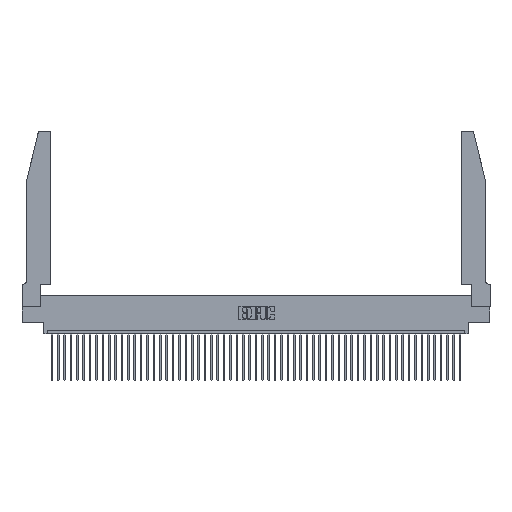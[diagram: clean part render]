
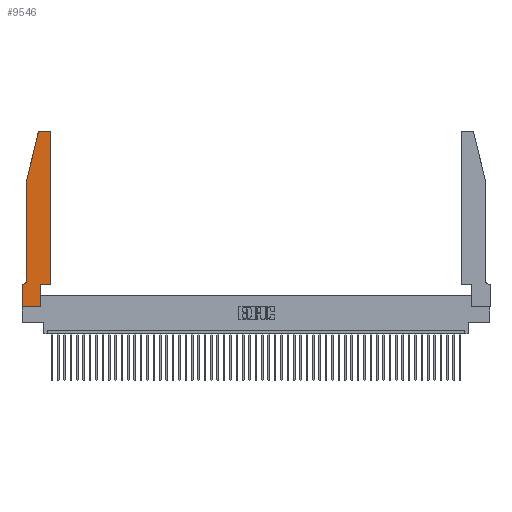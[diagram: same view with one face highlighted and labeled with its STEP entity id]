
A CAD part, top view. The second image highlights one B-rep face of the part: STEP entity #9546.
In plain terms, the highlighted planar face has unit normal (0, 0, 1).
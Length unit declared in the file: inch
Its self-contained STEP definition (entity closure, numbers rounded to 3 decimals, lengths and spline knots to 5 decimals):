
#22 = DIRECTION ( 'NONE',  ( 0., 1., 0. ) ) ;
#1451 = CARTESIAN_POINT ( 'NONE',  ( 0.0755, 2., 0.37 ) ) ;
#2126 = CARTESIAN_POINT ( 'NONE',  ( 0.25487, 2.72718, 0.37 ) ) ;
#3226 = CARTESIAN_POINT ( 'NONE',  ( 0.0755, 2., 0.37 ) ) ;
#3389 = EDGE_CURVE ( 'NONE', #45736, #35510, #20412, .T. ) ;
#4402 = CARTESIAN_POINT ( 'NONE',  ( 0.4205, 2.75, 0.37 ) ) ;
#4847 = DIRECTION ( 'NONE',  ( 0., -1., 0. ) ) ;
#5199 = ORIENTED_EDGE ( 'NONE', *, *, #43522, .T. ) ;
#6391 = DIRECTION ( 'NONE',  ( -1., 0., 0. ) ) ;
#7183 = DIRECTION ( 'NONE',  ( 1., 0., 0. ) ) ;
#8161 = VECTOR ( 'NONE', #22, 39.37008 ) ;
#8222 = VECTOR ( 'NONE', #27083, 39.37008 ) ;
#8641 = EDGE_LOOP ( 'NONE', ( #37591, #39959, #31837, #5199, #37440, #11541, #41976, #33160, #11432, #42461, #11227, #42321 ) ) ;
#8838 = EDGE_CURVE ( 'NONE', #35510, #29525, #29410, .T. ) ;
#9546 = ADVANCED_FACE ( 'NONE', ( #14076 ), #33500, .T. ) ;
#10850 = DIRECTION ( 'NONE',  ( -1., 0., 0. ) ) ;
#11227 = ORIENTED_EDGE ( 'NONE', *, *, #43294, .T. ) ;
#11432 = ORIENTED_EDGE ( 'NONE', *, *, #40064, .T. ) ;
#11541 = ORIENTED_EDGE ( 'NONE', *, *, #29513, .T. ) ;
#11752 = VERTEX_POINT ( 'NONE', #28298 ) ;
#12229 = DIRECTION ( 'NONE',  ( 1., 0., 0. ) ) ;
#12238 = EDGE_CURVE ( 'NONE', #29525, #23019, #36760, .T. ) ;
#12743 = DIRECTION ( 'NONE',  ( -0.239, -0.971, 0. ) ) ;
#13132 = VECTOR ( 'NONE', #14360, 39.37008 ) ;
#13478 = CARTESIAN_POINT ( 'NONE',  ( 0.2605, 2.75, 0.37 ) ) ;
#14076 = FACE_OUTER_BOUND ( 'NONE', #8641, .T. ) ;
#14146 = CARTESIAN_POINT ( 'NONE',  ( 0.2865, 0.35, 0.37 ) ) ;
#14197 = VECTOR ( 'NONE', #6391, 39.37008 ) ;
#14247 = VERTEX_POINT ( 'NONE', #35099 ) ;
#14360 = DIRECTION ( 'NONE',  ( 1., 0., 0. ) ) ;
#15518 = LINE ( 'NONE', #23782, #8161 ) ;
#15537 = VERTEX_POINT ( 'NONE', #40593 ) ;
#15557 = LINE ( 'NONE', #38149, #41897 ) ;
#15626 = LINE ( 'NONE', #42685, #8222 ) ;
#15811 = VERTEX_POINT ( 'NONE', #22862 ) ;
#16203 = VECTOR ( 'NONE', #4847, 39.37008 ) ;
#16302 = CARTESIAN_POINT ( 'NONE',  ( 0.284, 2.72, 0.37 ) ) ;
#17139 = EDGE_CURVE ( 'NONE', #15537, #23137, #50433, .T. ) ;
#20412 = LINE ( 'NONE', #13478, #40007 ) ;
#22862 = CARTESIAN_POINT ( 'NONE',  ( 0.0755, 0.42, 0.37 ) ) ;
#22872 = EDGE_CURVE ( 'NONE', #14247, #45736, #32179, .T. ) ;
#23019 = VERTEX_POINT ( 'NONE', #3226 ) ;
#23137 = VERTEX_POINT ( 'NONE', #27482 ) ;
#23782 = CARTESIAN_POINT ( 'NONE',  ( 0.2865, 0.35, 0.37 ) ) ;
#24404 = DIRECTION ( 'NONE',  ( 0., -1., 0. ) ) ;
#24999 = CARTESIAN_POINT ( 'NONE',  ( 0.0755, 2., 0.37 ) ) ;
#25021 = CIRCLE ( 'NONE', #38576, 0.07 ) ;
#25403 = DIRECTION ( 'NONE',  ( 1., 0., 0. ) ) ;
#26473 = VERTEX_POINT ( 'NONE', #37274 ) ;
#27083 = DIRECTION ( 'NONE',  ( 0., 1., 0. ) ) ;
#27482 = CARTESIAN_POINT ( 'NONE',  ( 0., 0., 0.37 ) ) ;
#27566 = VERTEX_POINT ( 'NONE', #30802 ) ;
#28298 = CARTESIAN_POINT ( 'NONE',  ( 0.4505, 0.35, 0.37 ) ) ;
#28463 = VERTEX_POINT ( 'NONE', #14146 ) ;
#29177 = DIRECTION ( 'NONE',  ( -1., 0., 0. ) ) ;
#29410 = CIRCLE ( 'NONE', #36288, 0.03 ) ;
#29513 = EDGE_CURVE ( 'NONE', #27566, #15537, #39858, .T. ) ;
#29525 = VERTEX_POINT ( 'NONE', #2126 ) ;
#29804 = CARTESIAN_POINT ( 'NONE',  ( 0.0755, 0.35, 0.37 ) ) ;
#30802 = CARTESIAN_POINT ( 'NONE',  ( 0.0055, 0.35, 0.37 ) ) ;
#31837 = ORIENTED_EDGE ( 'NONE', *, *, #12238, .T. ) ;
#32179 = CIRCLE ( 'NONE', #43151, 0.03 ) ;
#33160 = ORIENTED_EDGE ( 'NONE', *, *, #34089, .T. ) ;
#33500 = PLANE ( 'NONE',  #39182 ) ;
#33925 = DIRECTION ( 'NONE',  ( 0., 0., -1. ) ) ;
#34089 = EDGE_CURVE ( 'NONE', #23137, #26473, #15557, .T. ) ;
#34257 = CARTESIAN_POINT ( 'NONE',  ( 0.0055, 0.42, 0.37 ) ) ;
#34786 = DIRECTION ( 'NONE',  ( 1., 0., 0. ) ) ;
#35073 = CARTESIAN_POINT ( 'NONE',  ( 0., 0., 0.37 ) ) ;
#35099 = CARTESIAN_POINT ( 'NONE',  ( 0.4505, 2.72, 0.37 ) ) ;
#35510 = VERTEX_POINT ( 'NONE', #46935 ) ;
#35522 = VECTOR ( 'NONE', #12743, 39.37008 ) ;
#36288 = AXIS2_PLACEMENT_3D ( 'NONE', #16302, #40249, #12229 ) ;
#36760 = LINE ( 'NONE', #1451, #35522 ) ;
#37069 = DIRECTION ( 'NONE',  ( 0., 0., 1. ) ) ;
#37185 = CARTESIAN_POINT ( 'NONE',  ( 0.4205, 2.72, 0.37 ) ) ;
#37274 = CARTESIAN_POINT ( 'NONE',  ( 0.2865, 0., 0.37 ) ) ;
#37440 = ORIENTED_EDGE ( 'NONE', *, *, #46608, .T. ) ;
#37591 = ORIENTED_EDGE ( 'NONE', *, *, #3389, .T. ) ;
#38149 = CARTESIAN_POINT ( 'NONE',  ( 0., 0., 0.37 ) ) ;
#38268 = LINE ( 'NONE', #24999, #16203 ) ;
#38576 = AXIS2_PLACEMENT_3D ( 'NONE', #34257, #33925, #10850 ) ;
#39182 = AXIS2_PLACEMENT_3D ( 'NONE', #44745, #37069, #25403 ) ;
#39740 = EDGE_CURVE ( 'NONE', #28463, #11752, #44910, .T. ) ;
#39858 = LINE ( 'NONE', #29804, #14197 ) ;
#39959 = ORIENTED_EDGE ( 'NONE', *, *, #8838, .T. ) ;
#40007 = VECTOR ( 'NONE', #29177, 39.37008 ) ;
#40064 = EDGE_CURVE ( 'NONE', #26473, #28463, #15518, .T. ) ;
#40249 = DIRECTION ( 'NONE',  ( 0., 0., 1. ) ) ;
#40593 = CARTESIAN_POINT ( 'NONE',  ( 0., 0.35, 0.37 ) ) ;
#40961 = DIRECTION ( 'NONE',  ( 0., 0., 1. ) ) ;
#41897 = VECTOR ( 'NONE', #7183, 39.37008 ) ;
#41976 = ORIENTED_EDGE ( 'NONE', *, *, #17139, .T. ) ;
#42321 = ORIENTED_EDGE ( 'NONE', *, *, #22872, .T. ) ;
#42461 = ORIENTED_EDGE ( 'NONE', *, *, #39740, .T. ) ;
#42685 = CARTESIAN_POINT ( 'NONE',  ( 0.4505, 0.35, 0.37 ) ) ;
#43151 = AXIS2_PLACEMENT_3D ( 'NONE', #37185, #40961, #34786 ) ;
#43294 = EDGE_CURVE ( 'NONE', #11752, #14247, #15626, .T. ) ;
#43522 = EDGE_CURVE ( 'NONE', #23019, #15811, #38268, .T. ) ;
#43597 = VECTOR ( 'NONE', #24404, 39.37008 ) ;
#44745 = CARTESIAN_POINT ( 'NONE',  ( 0., 0.35, 0.37 ) ) ;
#44910 = LINE ( 'NONE', #45625, #13132 ) ;
#45625 = CARTESIAN_POINT ( 'NONE',  ( 0.4505, 0.35, 0.37 ) ) ;
#45736 = VERTEX_POINT ( 'NONE', #4402 ) ;
#46608 = EDGE_CURVE ( 'NONE', #15811, #27566, #25021, .T. ) ;
#46935 = CARTESIAN_POINT ( 'NONE',  ( 0.284, 2.75, 0.37 ) ) ;
#50433 = LINE ( 'NONE', #35073, #43597 ) ;
